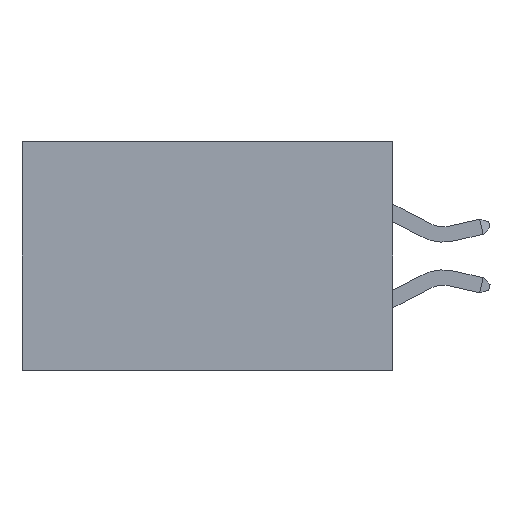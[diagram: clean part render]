
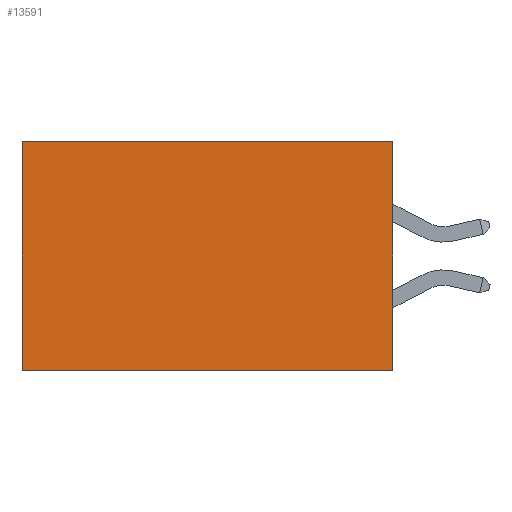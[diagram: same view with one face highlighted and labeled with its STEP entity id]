
A CAD part, left-side view. The second image highlights one B-rep face of the part: STEP entity #13591.
In plain terms, the highlighted planar face has unit normal (-1, 0, 0).
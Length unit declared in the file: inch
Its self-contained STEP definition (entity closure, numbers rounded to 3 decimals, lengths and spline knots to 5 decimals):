
#184 = LINE ( 'NONE', #22250, #16759 ) ;
#564 = VERTEX_POINT ( 'NONE', #12232 ) ;
#745 = DIRECTION ( 'NONE',  ( 0., 0., -1. ) ) ;
#924 = CARTESIAN_POINT ( 'NONE',  ( 0.2875, 0.6, 0. ) ) ;
#1383 = CARTESIAN_POINT ( 'NONE',  ( 0.2875, 0., 0. ) ) ;
#4586 = ORIENTED_EDGE ( 'NONE', *, *, #25819, .T. ) ;
#5569 = ORIENTED_EDGE ( 'NONE', *, *, #24636, .F. ) ;
#6192 = ORIENTED_EDGE ( 'NONE', *, *, #25144, .F. ) ;
#6853 = VERTEX_POINT ( 'NONE', #20536 ) ;
#7533 = VECTOR ( 'NONE', #745, 39.37008 ) ;
#8065 = VERTEX_POINT ( 'NONE', #14277 ) ;
#10974 = CARTESIAN_POINT ( 'NONE',  ( 0.2875, 0., 0. ) ) ;
#12232 = CARTESIAN_POINT ( 'NONE',  ( 0.2875, 0., -0.37 ) ) ;
#12766 = LINE ( 'NONE', #21626, #14369 ) ;
#13267 = VERTEX_POINT ( 'NONE', #1383 ) ;
#13591 = ADVANCED_FACE ( 'NONE', ( #17233 ), #23585, .F. ) ;
#13948 = AXIS2_PLACEMENT_3D ( 'NONE', #25709, #15553, #21959 ) ;
#13979 = EDGE_LOOP ( 'NONE', ( #4586, #6192, #5569, #20584 ) ) ;
#14277 = CARTESIAN_POINT ( 'NONE',  ( 0.2875, 0.6, 0. ) ) ;
#14369 = VECTOR ( 'NONE', #25916, 39.37008 ) ;
#15553 = DIRECTION ( 'NONE',  ( 1., 0., 0. ) ) ;
#15564 = EDGE_CURVE ( 'NONE', #13267, #8065, #184, .T. ) ;
#16382 = LINE ( 'NONE', #10974, #23631 ) ;
#16759 = VECTOR ( 'NONE', #24504, 39.37008 ) ;
#17148 = DIRECTION ( 'NONE',  ( 0., 0., -1. ) ) ;
#17233 = FACE_OUTER_BOUND ( 'NONE', #13979, .T. ) ;
#20536 = CARTESIAN_POINT ( 'NONE',  ( 0.2875, 0.6, -0.37 ) ) ;
#20584 = ORIENTED_EDGE ( 'NONE', *, *, #15564, .T. ) ;
#21626 = CARTESIAN_POINT ( 'NONE',  ( 0.2875, 0., -0.37 ) ) ;
#21959 = DIRECTION ( 'NONE',  ( 0., 0., -1. ) ) ;
#22250 = CARTESIAN_POINT ( 'NONE',  ( 0.2875, 0., 0. ) ) ;
#23585 = PLANE ( 'NONE',  #13948 ) ;
#23631 = VECTOR ( 'NONE', #17148, 39.37008 ) ;
#24504 = DIRECTION ( 'NONE',  ( 0., 1., 0. ) ) ;
#24539 = LINE ( 'NONE', #924, #7533 ) ;
#24636 = EDGE_CURVE ( 'NONE', #13267, #564, #16382, .T. ) ;
#25144 = EDGE_CURVE ( 'NONE', #564, #6853, #12766, .T. ) ;
#25709 = CARTESIAN_POINT ( 'NONE',  ( 0.2875, 0., 0. ) ) ;
#25819 = EDGE_CURVE ( 'NONE', #8065, #6853, #24539, .T. ) ;
#25916 = DIRECTION ( 'NONE',  ( 0., 1., 0. ) ) ;
